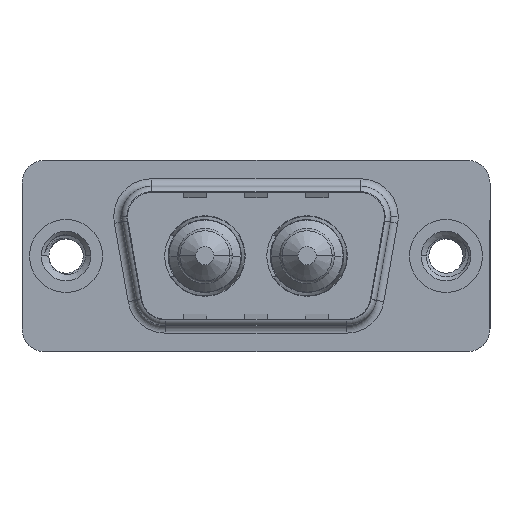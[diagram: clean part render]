
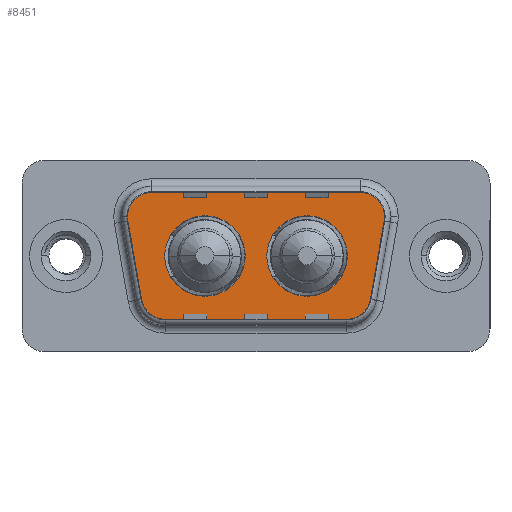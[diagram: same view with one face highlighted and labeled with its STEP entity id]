
A CAD part, top view. The second image highlights one B-rep face of the part: STEP entity #8451.
In plain terms, the highlighted planar face has unit normal (0, 0, 1).
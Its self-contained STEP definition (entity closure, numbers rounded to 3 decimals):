
#199 = VERTEX_POINT ( 'NONE', #6859 ) ;
#347 = VERTEX_POINT ( 'NONE', #9783 ) ;
#377 = ORIENTED_EDGE ( 'NONE', *, *, #6955, .T. ) ;
#406 = EDGE_CURVE ( 'NONE', #9537, #7105, #10737, .T. ) ;
#503 = DIRECTION ( 'NONE',  ( 0., 0., 1. ) ) ;
#748 = VERTEX_POINT ( 'NONE', #12730 ) ;
#839 = VERTEX_POINT ( 'NONE', #3757 ) ;
#955 = DIRECTION ( 'NONE',  ( 0., 0., 1. ) ) ;
#969 = LINE ( 'NONE', #12746, #6266 ) ;
#1007 = CARTESIAN_POINT ( 'NONE',  ( 5.436, 2.9, 0. ) ) ;
#1041 = DIRECTION ( 'NONE',  ( 1., 0., 0. ) ) ;
#1423 = VERTEX_POINT ( 'NONE', #3924 ) ;
#1532 = VERTEX_POINT ( 'NONE', #2562 ) ;
#1622 = DIRECTION ( 'NONE',  ( 0., 0., 1. ) ) ;
#1700 = EDGE_LOOP ( 'NONE', ( #13344, #2089 ) ) ;
#1957 = DIRECTION ( 'NONE',  ( 0., 0., 1. ) ) ;
#1962 = ORIENTED_EDGE ( 'NONE', *, *, #9617, .T. ) ;
#1995 = EDGE_CURVE ( 'NONE', #5880, #748, #9516, .T. ) ;
#2089 = ORIENTED_EDGE ( 'NONE', *, *, #6286, .F. ) ;
#2097 = DIRECTION ( 'NONE',  ( 1., 0., 0. ) ) ;
#2119 = CARTESIAN_POINT ( 'NONE',  ( 18.541, -2.9, 0. ) ) ;
#2319 = DIRECTION ( 'NONE',  ( 0., 0., 1. ) ) ;
#2562 = CARTESIAN_POINT ( 'NONE',  ( 21.564, 2.9, 0. ) ) ;
#2686 = EDGE_CURVE ( 'NONE', #839, #199, #10349, .T. ) ;
#2987 = CIRCLE ( 'NONE', #7299, 2. ) ;
#3016 = CARTESIAN_POINT ( 'NONE',  ( 18.541, -2.9, 0. ) ) ;
#3028 = DIRECTION ( 'NONE',  ( -1., 0., 0. ) ) ;
#3075 = FACE_BOUND ( 'NONE', #1700, .T. ) ;
#3132 = DIRECTION ( 'NONE',  ( 1., 0., 0. ) ) ;
#3161 = EDGE_CURVE ( 'NONE', #1532, #4073, #6086, .T. ) ;
#3529 = CARTESIAN_POINT ( 'NONE',  ( 6.459, -4.9, 0. ) ) ;
#3757 = CARTESIAN_POINT ( 'NONE',  ( 6.49, 0., 0. ) ) ;
#3758 = ORIENTED_EDGE ( 'NONE', *, *, #4005, .F. ) ;
#3889 = AXIS2_PLACEMENT_3D ( 'NONE', #3973, #3959, #3925 ) ;
#3924 = CARTESIAN_POINT ( 'NONE',  ( 6.459, -4.9, 0. ) ) ;
#3925 = DIRECTION ( 'NONE',  ( 1., 0., 0. ) ) ;
#3959 = DIRECTION ( 'NONE',  ( 0., 0., 1. ) ) ;
#3973 = CARTESIAN_POINT ( 'NONE',  ( 15.86, 0., 0. ) ) ;
#4005 = EDGE_CURVE ( 'NONE', #199, #839, #7605, .T. ) ;
#4073 = VERTEX_POINT ( 'NONE', #8263 ) ;
#4220 = AXIS2_PLACEMENT_3D ( 'NONE', #10381, #2319, #9185 ) ;
#4545 = CARTESIAN_POINT ( 'NONE',  ( 18.51, 0., 0. ) ) ;
#4728 = VERTEX_POINT ( 'NONE', #8720 ) ;
#4874 = AXIS2_PLACEMENT_3D ( 'NONE', #2119, #1957, #10943 ) ;
#5375 = VECTOR ( 'NONE', #1041, 1000. ) ;
#5461 = CARTESIAN_POINT ( 'NONE',  ( 13.21, 0., 0. ) ) ;
#5581 = AXIS2_PLACEMENT_3D ( 'NONE', #13413, #503, #12716 ) ;
#5757 = ORIENTED_EDGE ( 'NONE', *, *, #1995, .T. ) ;
#5793 = EDGE_CURVE ( 'NONE', #1423, #13159, #13858, .T. ) ;
#5862 = FACE_OUTER_BOUND ( 'NONE', #12278, .T. ) ;
#5880 = VERTEX_POINT ( 'NONE', #7325 ) ;
#6048 = EDGE_CURVE ( 'NONE', #13159, #9701, #11350, .T. ) ;
#6086 = CIRCLE ( 'NONE', #4220, 2. ) ;
#6160 = DIRECTION ( 'NONE',  ( 1., 0., 0. ) ) ;
#6266 = VECTOR ( 'NONE', #3028, 1000. ) ;
#6286 = EDGE_CURVE ( 'NONE', #7105, #9537, #11506, .T. ) ;
#6846 = CARTESIAN_POINT ( 'NONE',  ( 21.534, 2.553, 0. ) ) ;
#6859 = CARTESIAN_POINT ( 'NONE',  ( 11.79, 0., 0. ) ) ;
#6955 = EDGE_CURVE ( 'NONE', #4728, #5880, #9259, .T. ) ;
#7105 = VERTEX_POINT ( 'NONE', #5461 ) ;
#7299 = AXIS2_PLACEMENT_3D ( 'NONE', #8016, #1622, #9123 ) ;
#7325 = CARTESIAN_POINT ( 'NONE',  ( 3.466, 2.553, 0. ) ) ;
#7329 = CARTESIAN_POINT ( 'NONE',  ( 6.459, -2.9, 0. ) ) ;
#7605 = CIRCLE ( 'NONE', #5581, 2.65 ) ;
#7883 = AXIS2_PLACEMENT_3D ( 'NONE', #1007, #8476, #2097 ) ;
#7947 = DIRECTION ( 'NONE',  ( 0.174, 0.985, 0. ) ) ;
#8016 = CARTESIAN_POINT ( 'NONE',  ( 19.564, 2.9, 0. ) ) ;
#8263 = CARTESIAN_POINT ( 'NONE',  ( 19.564, 4.9, 0. ) ) ;
#8426 = DIRECTION ( 'NONE',  ( -1., 0., 0. ) ) ;
#8451 = ADVANCED_FACE ( 'NONE', ( #3075, #8736, #5862 ), #9375, .T. ) ;
#8476 = DIRECTION ( 'NONE',  ( 0., 0., 1. ) ) ;
#8720 = CARTESIAN_POINT ( 'NONE',  ( 5.436, 4.9, 0. ) ) ;
#8736 = FACE_BOUND ( 'NONE', #11796, .T. ) ;
#8979 = ORIENTED_EDGE ( 'NONE', *, *, #11652, .T. ) ;
#9123 = DIRECTION ( 'NONE',  ( -1., 0., 0. ) ) ;
#9185 = DIRECTION ( 'NONE',  ( -1., 0., 0. ) ) ;
#9259 = CIRCLE ( 'NONE', #7883, 2. ) ;
#9375 = PLANE ( 'NONE',  #9713 ) ;
#9516 = LINE ( 'NONE', #10996, #11761 ) ;
#9537 = VERTEX_POINT ( 'NONE', #4545 ) ;
#9617 = EDGE_CURVE ( 'NONE', #9701, #347, #10082, .T. ) ;
#9648 = DIRECTION ( 'NONE',  ( 0.174, -0.985, 0. ) ) ;
#9701 = VERTEX_POINT ( 'NONE', #12453 ) ;
#9713 = AXIS2_PLACEMENT_3D ( 'NONE', #3016, #12788, #6160 ) ;
#9783 = CARTESIAN_POINT ( 'NONE',  ( 21.534, 2.553, 0. ) ) ;
#9839 = ORIENTED_EDGE ( 'NONE', *, *, #6048, .T. ) ;
#9881 = DIRECTION ( 'NONE',  ( 1., 0., 0. ) ) ;
#10082 = LINE ( 'NONE', #6846, #12724 ) ;
#10349 = CIRCLE ( 'NONE', #12185, 2.65 ) ;
#10381 = CARTESIAN_POINT ( 'NONE',  ( 19.564, 2.9, 0. ) ) ;
#10553 = CARTESIAN_POINT ( 'NONE',  ( 15.86, 0., 0. ) ) ;
#10648 = AXIS2_PLACEMENT_3D ( 'NONE', #7329, #955, #8426 ) ;
#10656 = CARTESIAN_POINT ( 'NONE',  ( 9.14, 0., 0. ) ) ;
#10737 = CIRCLE ( 'NONE', #12928, 2.65 ) ;
#10860 = ORIENTED_EDGE ( 'NONE', *, *, #3161, .T. ) ;
#10943 = DIRECTION ( 'NONE',  ( 1., 0., 0. ) ) ;
#10996 = CARTESIAN_POINT ( 'NONE',  ( 3.466, 2.553, 0. ) ) ;
#11350 = CIRCLE ( 'NONE', #4874, 2. ) ;
#11506 = CIRCLE ( 'NONE', #3889, 2.65 ) ;
#11648 = DIRECTION ( 'NONE',  ( 0., 0., 1. ) ) ;
#11652 = EDGE_CURVE ( 'NONE', #748, #1423, #14136, .T. ) ;
#11739 = ORIENTED_EDGE ( 'NONE', *, *, #2686, .F. ) ;
#11761 = VECTOR ( 'NONE', #9648, 1000. ) ;
#11796 = EDGE_LOOP ( 'NONE', ( #3758, #11739 ) ) ;
#11939 = ORIENTED_EDGE ( 'NONE', *, *, #5793, .T. ) ;
#12089 = CARTESIAN_POINT ( 'NONE',  ( 18.541, -4.9, 0. ) ) ;
#12143 = EDGE_CURVE ( 'NONE', #4073, #4728, #969, .T. ) ;
#12185 = AXIS2_PLACEMENT_3D ( 'NONE', #10656, #13776, #9881 ) ;
#12278 = EDGE_LOOP ( 'NONE', ( #9839, #1962, #13555, #10860, #14263, #377, #5757, #8979, #11939 ) ) ;
#12453 = CARTESIAN_POINT ( 'NONE',  ( 20.511, -3.247, 0. ) ) ;
#12716 = DIRECTION ( 'NONE',  ( 1., 0., 0. ) ) ;
#12724 = VECTOR ( 'NONE', #7947, 1000. ) ;
#12730 = CARTESIAN_POINT ( 'NONE',  ( 4.489, -3.247, 0. ) ) ;
#12746 = CARTESIAN_POINT ( 'NONE',  ( 5.436, 4.9, 0. ) ) ;
#12788 = DIRECTION ( 'NONE',  ( 0., 0., 1. ) ) ;
#12928 = AXIS2_PLACEMENT_3D ( 'NONE', #10553, #11648, #3132 ) ;
#13159 = VERTEX_POINT ( 'NONE', #12089 ) ;
#13321 = EDGE_CURVE ( 'NONE', #347, #1532, #2987, .T. ) ;
#13344 = ORIENTED_EDGE ( 'NONE', *, *, #406, .F. ) ;
#13413 = CARTESIAN_POINT ( 'NONE',  ( 9.14, 0., 0. ) ) ;
#13555 = ORIENTED_EDGE ( 'NONE', *, *, #13321, .T. ) ;
#13776 = DIRECTION ( 'NONE',  ( 0., 0., 1. ) ) ;
#13858 = LINE ( 'NONE', #3529, #5375 ) ;
#14136 = CIRCLE ( 'NONE', #10648, 2. ) ;
#14263 = ORIENTED_EDGE ( 'NONE', *, *, #12143, .T. ) ;
